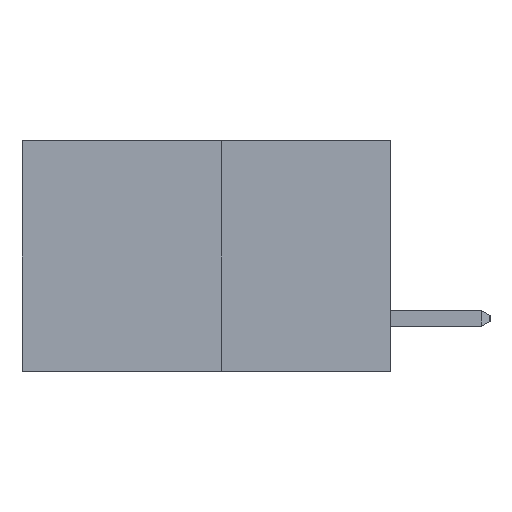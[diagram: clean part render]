
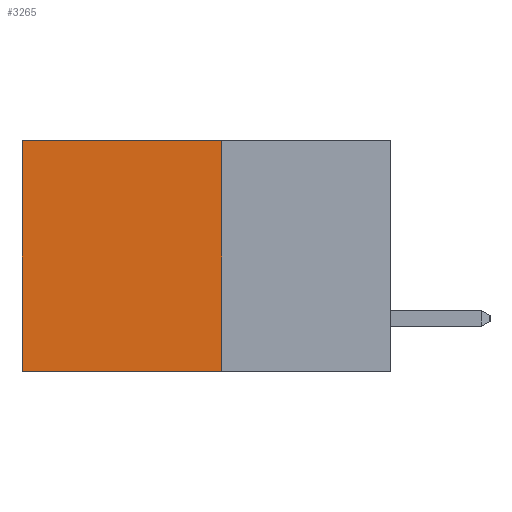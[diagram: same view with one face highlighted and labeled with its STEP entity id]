
A CAD part, left-side view. The second image highlights one B-rep face of the part: STEP entity #3265.
In plain terms, the highlighted planar face has unit normal (-1, 0, 0).
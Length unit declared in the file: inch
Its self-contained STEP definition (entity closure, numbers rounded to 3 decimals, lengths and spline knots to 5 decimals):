
#664 = DIRECTION ( 'NONE',  ( 0., 0., -1. ) ) ;
#1014 = CARTESIAN_POINT ( 'NONE',  ( 0.277, 0.59, -0.37 ) ) ;
#1235 = DIRECTION ( 'NONE',  ( 1., 0., 0. ) ) ;
#1329 = ORIENTED_EDGE ( 'NONE', *, *, #17987, .T. ) ;
#1950 = VERTEX_POINT ( 'NONE', #13371 ) ;
#2170 = DIRECTION ( 'NONE',  ( 0., 0., -1. ) ) ;
#3265 = ADVANCED_FACE ( 'NONE', ( #8264 ), #17712, .F. ) ;
#3286 = EDGE_CURVE ( 'NONE', #10013, #7665, #19761, .T. ) ;
#3587 = VECTOR ( 'NONE', #15793, 39.37008 ) ;
#3695 = VECTOR ( 'NONE', #2170, 39.37008 ) ;
#3759 = EDGE_CURVE ( 'NONE', #7665, #6257, #19294, .T. ) ;
#4181 = LINE ( 'NONE', #5225, #3695 ) ;
#4945 = CARTESIAN_POINT ( 'NONE',  ( 0.277, 0.27, 0. ) ) ;
#5225 = CARTESIAN_POINT ( 'NONE',  ( 0.277, 0.59, -0.37 ) ) ;
#5890 = DIRECTION ( 'NONE',  ( 0., 1., 0. ) ) ;
#5993 = CARTESIAN_POINT ( 'NONE',  ( 0.277, 0.27, 0. ) ) ;
#6087 = EDGE_CURVE ( 'NONE', #10013, #1950, #9421, .T. ) ;
#6257 = VERTEX_POINT ( 'NONE', #1014 ) ;
#7220 = AXIS2_PLACEMENT_3D ( 'NONE', #10172, #1235, #18109 ) ;
#7665 = VERTEX_POINT ( 'NONE', #17484 ) ;
#8264 = FACE_OUTER_BOUND ( 'NONE', #11690, .T. ) ;
#9421 = LINE ( 'NONE', #5993, #16997 ) ;
#10013 = VERTEX_POINT ( 'NONE', #4945 ) ;
#10172 = CARTESIAN_POINT ( 'NONE',  ( 0.277, 0.27, -0.37 ) ) ;
#11690 = EDGE_LOOP ( 'NONE', ( #1329, #14611, #13394, #13894 ) ) ;
#13371 = CARTESIAN_POINT ( 'NONE',  ( 0.277, 0.59, 0. ) ) ;
#13394 = ORIENTED_EDGE ( 'NONE', *, *, #3286, .F. ) ;
#13894 = ORIENTED_EDGE ( 'NONE', *, *, #6087, .T. ) ;
#14030 = CARTESIAN_POINT ( 'NONE',  ( 0.277, 0.27, -0.37 ) ) ;
#14611 = ORIENTED_EDGE ( 'NONE', *, *, #3759, .F. ) ;
#15376 = VECTOR ( 'NONE', #664, 39.37008 ) ;
#15793 = DIRECTION ( 'NONE',  ( 0., 1., 0. ) ) ;
#16997 = VECTOR ( 'NONE', #5890, 39.37008 ) ;
#17358 = CARTESIAN_POINT ( 'NONE',  ( 0.277, 0.27, -0.37 ) ) ;
#17484 = CARTESIAN_POINT ( 'NONE',  ( 0.277, 0.27, -0.37 ) ) ;
#17712 = PLANE ( 'NONE',  #7220 ) ;
#17987 = EDGE_CURVE ( 'NONE', #1950, #6257, #4181, .T. ) ;
#18109 = DIRECTION ( 'NONE',  ( 0., 0., -1. ) ) ;
#19294 = LINE ( 'NONE', #14030, #3587 ) ;
#19761 = LINE ( 'NONE', #17358, #15376 ) ;
